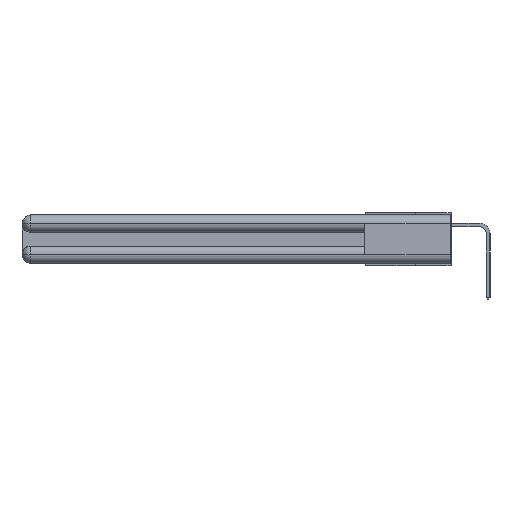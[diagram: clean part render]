
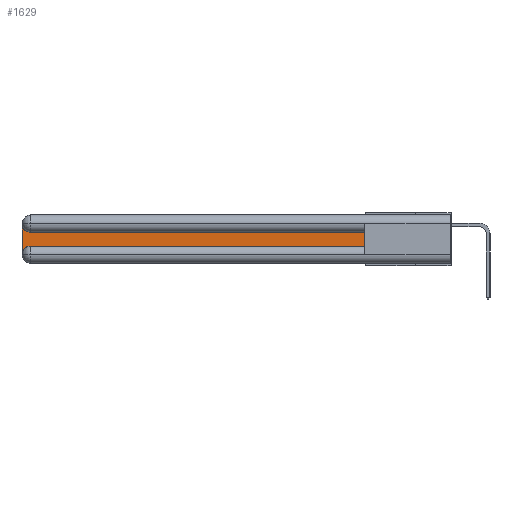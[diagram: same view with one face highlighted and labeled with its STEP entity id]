
A CAD part, left-side view. The second image highlights one B-rep face of the part: STEP entity #1629.
In plain terms, the highlighted planar face has unit normal (-1, 0, 0).
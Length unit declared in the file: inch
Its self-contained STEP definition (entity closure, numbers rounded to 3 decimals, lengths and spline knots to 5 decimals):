
#1629 = ADVANCED_FACE ( 'NONE', ( #5321 ), #34448, .F. ) ;
#2275 = ORIENTED_EDGE ( 'NONE', *, *, #23652, .T. ) ;
#2285 = CARTESIAN_POINT ( 'NONE',  ( 0.075, 0.6, -0.1225 ) ) ;
#4797 = EDGE_CURVE ( 'NONE', #23521, #10171, #33628, .T. ) ;
#4814 = LINE ( 'NONE', #18766, #14016 ) ;
#5172 = DIRECTION ( 'NONE',  ( 1., 0., 0. ) ) ;
#5321 = FACE_OUTER_BOUND ( 'NONE', #8247, .T. ) ;
#5453 = DIRECTION ( 'NONE',  ( 0., 0., 1. ) ) ;
#6270 = VERTEX_POINT ( 'NONE', #17648 ) ;
#6345 = CIRCLE ( 'NONE', #31583, 0.06 ) ;
#7425 = CARTESIAN_POINT ( 'NONE',  ( 0.075, 3., -0.1225 ) ) ;
#7531 = DIRECTION ( 'NONE',  ( 1., 0., 0. ) ) ;
#8247 = EDGE_LOOP ( 'NONE', ( #31611, #23901, #12510, #32336, #28839, #2275 ) ) ;
#8784 = VERTEX_POINT ( 'NONE', #2285 ) ;
#9531 = AXIS2_PLACEMENT_3D ( 'NONE', #7425, #7531, #18486 ) ;
#10159 = LINE ( 'NONE', #29130, #30631 ) ;
#10171 = VERTEX_POINT ( 'NONE', #32552 ) ;
#10175 = EDGE_CURVE ( 'NONE', #20580, #6270, #13493, .T. ) ;
#10688 = DIRECTION ( 'NONE',  ( 0., 0., -1. ) ) ;
#12510 = ORIENTED_EDGE ( 'NONE', *, *, #4797, .T. ) ;
#13493 = LINE ( 'NONE', #13891, #19766 ) ;
#13891 = CARTESIAN_POINT ( 'NONE',  ( 0.075, 0.6, -0.2175 ) ) ;
#14016 = VECTOR ( 'NONE', #5453, 39.37008 ) ;
#15444 = EDGE_CURVE ( 'NONE', #8784, #20665, #10159, .T. ) ;
#15521 = EDGE_CURVE ( 'NONE', #10171, #20580, #18937, .T. ) ;
#16166 = CARTESIAN_POINT ( 'NONE',  ( 0.075, 2.94, -0.2775 ) ) ;
#17648 = CARTESIAN_POINT ( 'NONE',  ( 0.075, 0.6, -0.2175 ) ) ;
#18486 = DIRECTION ( 'NONE',  ( 0., 0., -1. ) ) ;
#18766 = CARTESIAN_POINT ( 'NONE',  ( 0.075, 0.6, -0.2175 ) ) ;
#18937 = CIRCLE ( 'NONE', #31184, 0.06 ) ;
#19177 = CARTESIAN_POINT ( 'NONE',  ( 0.075, 2.94, -0.1225 ) ) ;
#19461 = VECTOR ( 'NONE', #22866, 39.37008 ) ;
#19766 = VECTOR ( 'NONE', #27316, 39.37008 ) ;
#20378 = CARTESIAN_POINT ( 'NONE',  ( 0.075, 3., -0.0625 ) ) ;
#20580 = VERTEX_POINT ( 'NONE', #29350 ) ;
#20665 = VERTEX_POINT ( 'NONE', #19177 ) ;
#20942 = DIRECTION ( 'NONE',  ( 0., 1., 0. ) ) ;
#22866 = DIRECTION ( 'NONE',  ( 0., 0., -1. ) ) ;
#23152 = DIRECTION ( 'NONE',  ( 1., 0., 0. ) ) ;
#23521 = VERTEX_POINT ( 'NONE', #20378 ) ;
#23652 = EDGE_CURVE ( 'NONE', #6270, #8784, #4814, .T. ) ;
#23901 = ORIENTED_EDGE ( 'NONE', *, *, #25722, .T. ) ;
#25557 = CARTESIAN_POINT ( 'NONE',  ( 0.075, 3., -0.2175 ) ) ;
#25722 = EDGE_CURVE ( 'NONE', #20665, #23521, #6345, .T. ) ;
#27316 = DIRECTION ( 'NONE',  ( 0., -1., 0. ) ) ;
#28745 = CARTESIAN_POINT ( 'NONE',  ( 0.075, 2.94, -0.0625 ) ) ;
#28839 = ORIENTED_EDGE ( 'NONE', *, *, #10175, .T. ) ;
#29130 = CARTESIAN_POINT ( 'NONE',  ( 0.075, 0.6, -0.1225 ) ) ;
#29350 = CARTESIAN_POINT ( 'NONE',  ( 0.075, 2.94, -0.2175 ) ) ;
#30631 = VECTOR ( 'NONE', #20942, 39.37008 ) ;
#31184 = AXIS2_PLACEMENT_3D ( 'NONE', #16166, #5172, #10688 ) ;
#31294 = DIRECTION ( 'NONE',  ( 0., 0., -1. ) ) ;
#31583 = AXIS2_PLACEMENT_3D ( 'NONE', #28745, #23152, #31294 ) ;
#31611 = ORIENTED_EDGE ( 'NONE', *, *, #15444, .T. ) ;
#32336 = ORIENTED_EDGE ( 'NONE', *, *, #15521, .T. ) ;
#32552 = CARTESIAN_POINT ( 'NONE',  ( 0.075, 3., -0.2775 ) ) ;
#33628 = LINE ( 'NONE', #25557, #19461 ) ;
#34448 = PLANE ( 'NONE',  #9531 ) ;
